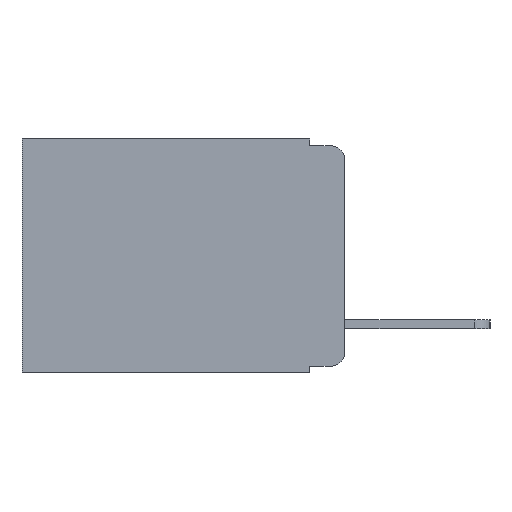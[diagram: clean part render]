
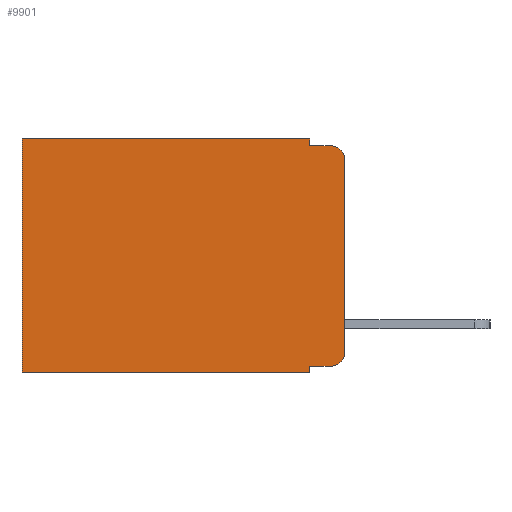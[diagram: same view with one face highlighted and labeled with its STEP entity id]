
A CAD part, left-side view. The second image highlights one B-rep face of the part: STEP entity #9901.
In plain terms, the highlighted planar face has unit normal (-1, 0, 0).
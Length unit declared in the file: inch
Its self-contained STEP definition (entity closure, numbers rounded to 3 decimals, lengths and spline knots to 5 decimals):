
#154 = EDGE_CURVE ( 'NONE', #1413, #3225, #205, .T. ) ;
#205 = LINE ( 'NONE', #10841, #2455 ) ;
#226 = LINE ( 'NONE', #1314, #6821 ) ;
#346 = DIRECTION ( 'NONE',  ( 0., 0., -1. ) ) ;
#404 = CARTESIAN_POINT ( 'NONE',  ( 0.298, 0.051, 0. ) ) ;
#624 = CARTESIAN_POINT ( 'NONE',  ( 0.298, 0.051, -0.01 ) ) ;
#639 = AXIS2_PLACEMENT_3D ( 'NONE', #7807, #2613, #8651 ) ;
#734 = CARTESIAN_POINT ( 'NONE',  ( 0.298, 0.051, -0.333 ) ) ;
#909 = VERTEX_POINT ( 'NONE', #4844 ) ;
#1106 = PLANE ( 'NONE',  #6710 ) ;
#1119 = LINE ( 'NONE', #4164, #5443 ) ;
#1192 = DIRECTION ( 'NONE',  ( 0., -1., 0. ) ) ;
#1314 = CARTESIAN_POINT ( 'NONE',  ( 0.298, 0.051, -0.333 ) ) ;
#1342 = CARTESIAN_POINT ( 'NONE',  ( 0.298, 0.051, 0. ) ) ;
#1413 = VERTEX_POINT ( 'NONE', #7651 ) ;
#1450 = VERTEX_POINT ( 'NONE', #6176 ) ;
#1698 = ORIENTED_EDGE ( 'NONE', *, *, #8786, .T. ) ;
#1710 = EDGE_CURVE ( 'NONE', #7643, #3225, #7061, .T. ) ;
#2455 = VECTOR ( 'NONE', #10093, 39.37008 ) ;
#2471 = VECTOR ( 'NONE', #3252, 39.37008 ) ;
#2481 = CIRCLE ( 'NONE', #639, 0.02 ) ;
#2613 = DIRECTION ( 'NONE',  ( -1., 0., 0. ) ) ;
#2739 = ORIENTED_EDGE ( 'NONE', *, *, #10881, .F. ) ;
#2811 = CARTESIAN_POINT ( 'NONE',  ( 0.298, 0., 0. ) ) ;
#3031 = ORIENTED_EDGE ( 'NONE', *, *, #1710, .T. ) ;
#3067 = EDGE_CURVE ( 'NONE', #3382, #8120, #9307, .T. ) ;
#3149 = LINE ( 'NONE', #624, #7231 ) ;
#3169 = ORIENTED_EDGE ( 'NONE', *, *, #3871, .F. ) ;
#3225 = VERTEX_POINT ( 'NONE', #10715 ) ;
#3252 = DIRECTION ( 'NONE',  ( 0., 1., 0. ) ) ;
#3382 = VERTEX_POINT ( 'NONE', #734 ) ;
#3574 = ORIENTED_EDGE ( 'NONE', *, *, #5975, .T. ) ;
#3871 = EDGE_CURVE ( 'NONE', #1450, #909, #10557, .T. ) ;
#4164 = CARTESIAN_POINT ( 'NONE',  ( 0.298, 0., -0.343 ) ) ;
#4570 = DIRECTION ( 'NONE',  ( 1., 0., 0. ) ) ;
#4666 = VECTOR ( 'NONE', #9787, 39.37008 ) ;
#4675 = ORIENTED_EDGE ( 'NONE', *, *, #9037, .T. ) ;
#4844 = CARTESIAN_POINT ( 'NONE',  ( 0.298, 0.051, -0.01 ) ) ;
#4933 = LINE ( 'NONE', #7324, #4666 ) ;
#5357 = AXIS2_PLACEMENT_3D ( 'NONE', #6336, #5929, #9518 ) ;
#5443 = VECTOR ( 'NONE', #8489, 39.37008 ) ;
#5628 = EDGE_CURVE ( 'NONE', #909, #7993, #3149, .T. ) ;
#5632 = CARTESIAN_POINT ( 'NONE',  ( 0.298, 0.473, 0. ) ) ;
#5826 = CARTESIAN_POINT ( 'NONE',  ( 0.298, 0.051, -0.343 ) ) ;
#5850 = VECTOR ( 'NONE', #10462, 39.37008 ) ;
#5929 = DIRECTION ( 'NONE',  ( -1., 0., 0. ) ) ;
#5975 = EDGE_CURVE ( 'NONE', #3382, #7643, #226, .T. ) ;
#6176 = CARTESIAN_POINT ( 'NONE',  ( 0.298, 0.051, 0. ) ) ;
#6336 = CARTESIAN_POINT ( 'NONE',  ( 0.298, 0.02, -0.313 ) ) ;
#6710 = AXIS2_PLACEMENT_3D ( 'NONE', #2811, #4570, #10474 ) ;
#6821 = VECTOR ( 'NONE', #10061, 39.37008 ) ;
#7061 = CIRCLE ( 'NONE', #5357, 0.02 ) ;
#7098 = VECTOR ( 'NONE', #346, 39.37008 ) ;
#7231 = VECTOR ( 'NONE', #1192, 39.37008 ) ;
#7324 = CARTESIAN_POINT ( 'NONE',  ( 0.298, 0.473, 0. ) ) ;
#7375 = FACE_OUTER_BOUND ( 'NONE', #9001, .T. ) ;
#7643 = VERTEX_POINT ( 'NONE', #7823 ) ;
#7651 = CARTESIAN_POINT ( 'NONE',  ( 0.298, 0., -0.03 ) ) ;
#7807 = CARTESIAN_POINT ( 'NONE',  ( 0.298, 0.02, -0.03 ) ) ;
#7823 = CARTESIAN_POINT ( 'NONE',  ( 0.298, 0.02, -0.333 ) ) ;
#7890 = ORIENTED_EDGE ( 'NONE', *, *, #9224, .T. ) ;
#7993 = VERTEX_POINT ( 'NONE', #10693 ) ;
#8095 = ORIENTED_EDGE ( 'NONE', *, *, #3067, .F. ) ;
#8120 = VERTEX_POINT ( 'NONE', #5826 ) ;
#8489 = DIRECTION ( 'NONE',  ( 0., 1., 0. ) ) ;
#8644 = CARTESIAN_POINT ( 'NONE',  ( 0.298, 0.473, -0.343 ) ) ;
#8651 = DIRECTION ( 'NONE',  ( 0., 0., -1. ) ) ;
#8786 = EDGE_CURVE ( 'NONE', #1413, #7993, #2481, .T. ) ;
#9001 = EDGE_LOOP ( 'NONE', ( #10745, #1698, #9560, #3169, #7890, #4675, #2739, #8095, #3574, #3031 ) ) ;
#9037 = EDGE_CURVE ( 'NONE', #10667, #9777, #4933, .T. ) ;
#9224 = EDGE_CURVE ( 'NONE', #1450, #10667, #9309, .T. ) ;
#9307 = LINE ( 'NONE', #404, #7098 ) ;
#9309 = LINE ( 'NONE', #10853, #2471 ) ;
#9518 = DIRECTION ( 'NONE',  ( 0., 0., -1. ) ) ;
#9560 = ORIENTED_EDGE ( 'NONE', *, *, #5628, .F. ) ;
#9777 = VERTEX_POINT ( 'NONE', #8644 ) ;
#9787 = DIRECTION ( 'NONE',  ( 0., 0., -1. ) ) ;
#9901 = ADVANCED_FACE ( 'NONE', ( #7375 ), #1106, .F. ) ;
#10061 = DIRECTION ( 'NONE',  ( 0., -1., 0. ) ) ;
#10093 = DIRECTION ( 'NONE',  ( 0., 0., -1. ) ) ;
#10462 = DIRECTION ( 'NONE',  ( 0., 0., -1. ) ) ;
#10474 = DIRECTION ( 'NONE',  ( 0., 0., -1. ) ) ;
#10557 = LINE ( 'NONE', #1342, #5850 ) ;
#10667 = VERTEX_POINT ( 'NONE', #5632 ) ;
#10693 = CARTESIAN_POINT ( 'NONE',  ( 0.298, 0.02, -0.01 ) ) ;
#10715 = CARTESIAN_POINT ( 'NONE',  ( 0.298, 0., -0.313 ) ) ;
#10745 = ORIENTED_EDGE ( 'NONE', *, *, #154, .F. ) ;
#10841 = CARTESIAN_POINT ( 'NONE',  ( 0.298, 0., 0. ) ) ;
#10853 = CARTESIAN_POINT ( 'NONE',  ( 0.298, 0., 0. ) ) ;
#10881 = EDGE_CURVE ( 'NONE', #8120, #9777, #1119, .T. ) ;
